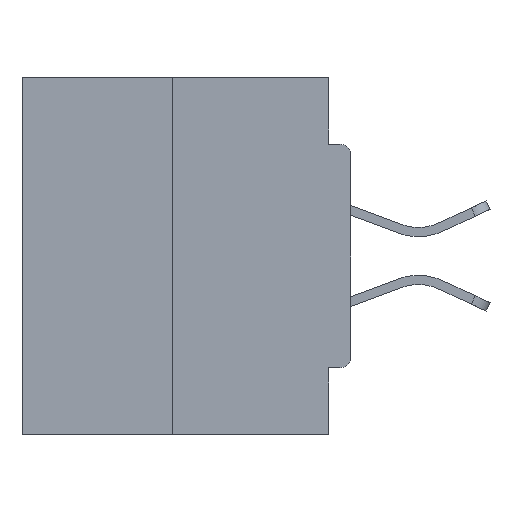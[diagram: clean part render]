
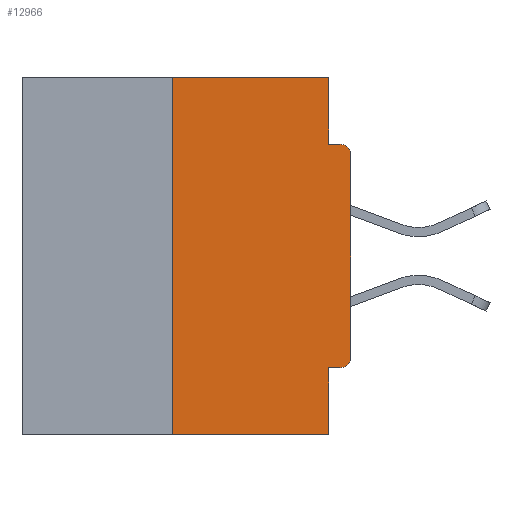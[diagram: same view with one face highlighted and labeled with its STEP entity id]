
A CAD part, left-side view. The second image highlights one B-rep face of the part: STEP entity #12966.
In plain terms, the highlighted planar face has unit normal (-1, 0, 0).
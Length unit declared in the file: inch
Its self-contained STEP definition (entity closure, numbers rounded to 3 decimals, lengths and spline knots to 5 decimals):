
#333 = VECTOR ( 'NONE', #12182, 39.37008 ) ;
#417 = CARTESIAN_POINT ( 'NONE',  ( 0., 0.015, -0.4065 ) ) ;
#547 = CARTESIAN_POINT ( 'NONE',  ( 0., 0., -0.1085 ) ) ;
#563 = EDGE_CURVE ( 'NONE', #22373, #10864, #4484, .T. ) ;
#643 = VERTEX_POINT ( 'NONE', #36403 ) ;
#2013 = VERTEX_POINT ( 'NONE', #417 ) ;
#2313 = CARTESIAN_POINT ( 'NONE',  ( 0., 0.25, 0. ) ) ;
#3175 = LINE ( 'NONE', #6130, #9970 ) ;
#3358 = CIRCLE ( 'NONE', #30537, 0.015 ) ;
#3450 = CARTESIAN_POINT ( 'NONE',  ( 0., 0., 0. ) ) ;
#3706 = EDGE_CURVE ( 'NONE', #19159, #22373, #3175, .T. ) ;
#4159 = VERTEX_POINT ( 'NONE', #19942 ) ;
#4265 = AXIS2_PLACEMENT_3D ( 'NONE', #24446, #10543, #18491 ) ;
#4347 = ORIENTED_EDGE ( 'NONE', *, *, #21684, .F. ) ;
#4484 = LINE ( 'NONE', #18696, #19884 ) ;
#5121 = CARTESIAN_POINT ( 'NONE',  ( 0., 0., -0.3915 ) ) ;
#5281 = DIRECTION ( 'NONE',  ( 0., 0., -1. ) ) ;
#6001 = VECTOR ( 'NONE', #30020, 39.37008 ) ;
#6130 = CARTESIAN_POINT ( 'NONE',  ( 0., 0.031, 0. ) ) ;
#6259 = VERTEX_POINT ( 'NONE', #2313 ) ;
#6501 = VERTEX_POINT ( 'NONE', #547 ) ;
#8288 = DIRECTION ( 'NONE',  ( 1., 0., 0. ) ) ;
#8590 = DIRECTION ( 'NONE',  ( -1., 0., 0. ) ) ;
#9970 = VECTOR ( 'NONE', #28150, 39.37008 ) ;
#10354 = DIRECTION ( 'NONE',  ( 0., -1., 0. ) ) ;
#10543 = DIRECTION ( 'NONE',  ( -1., 0., 0. ) ) ;
#10864 = VERTEX_POINT ( 'NONE', #24368 ) ;
#11917 = VECTOR ( 'NONE', #15080, 39.37008 ) ;
#12182 = DIRECTION ( 'NONE',  ( 0., 1., 0. ) ) ;
#12185 = VERTEX_POINT ( 'NONE', #5121 ) ;
#12966 = ADVANCED_FACE ( 'NONE', ( #22513 ), #30677, .F. ) ;
#13033 = VECTOR ( 'NONE', #10354, 39.37008 ) ;
#13165 = LINE ( 'NONE', #35702, #6001 ) ;
#14017 = CARTESIAN_POINT ( 'NONE',  ( 0., 0.031, 0. ) ) ;
#14531 = EDGE_CURVE ( 'NONE', #4159, #19015, #26332, .T. ) ;
#14701 = LINE ( 'NONE', #3450, #32940 ) ;
#15080 = DIRECTION ( 'NONE',  ( 0., -1., 0. ) ) ;
#15163 = LINE ( 'NONE', #34755, #333 ) ;
#15308 = CARTESIAN_POINT ( 'NONE',  ( 0., 0.031, -0.0935 ) ) ;
#18129 = EDGE_LOOP ( 'NONE', ( #18596, #4347, #33039, #26468, #20094, #22767, #28014, #28565, #25406, #29404 ) ) ;
#18254 = AXIS2_PLACEMENT_3D ( 'NONE', #28437, #8288, #33780 ) ;
#18403 = CARTESIAN_POINT ( 'NONE',  ( 0., 0.46, 0. ) ) ;
#18491 = DIRECTION ( 'NONE',  ( 0., 0., -1. ) ) ;
#18596 = ORIENTED_EDGE ( 'NONE', *, *, #24082, .F. ) ;
#18662 = CARTESIAN_POINT ( 'NONE',  ( 0., 0.031, -0.5 ) ) ;
#18696 = CARTESIAN_POINT ( 'NONE',  ( 0., 0., -0.0935 ) ) ;
#19015 = VERTEX_POINT ( 'NONE', #18662 ) ;
#19159 = VERTEX_POINT ( 'NONE', #14017 ) ;
#19709 = DIRECTION ( 'NONE',  ( 0., 0., 1. ) ) ;
#19884 = VECTOR ( 'NONE', #24459, 39.37008 ) ;
#19942 = CARTESIAN_POINT ( 'NONE',  ( 0., 0.031, -0.4065 ) ) ;
#20094 = ORIENTED_EDGE ( 'NONE', *, *, #33133, .F. ) ;
#20981 = EDGE_CURVE ( 'NONE', #12185, #6501, #14701, .T. ) ;
#21684 = EDGE_CURVE ( 'NONE', #643, #6259, #13165, .T. ) ;
#22123 = EDGE_CURVE ( 'NONE', #643, #19015, #24247, .T. ) ;
#22373 = VERTEX_POINT ( 'NONE', #15308 ) ;
#22513 = FACE_OUTER_BOUND ( 'NONE', #18129, .T. ) ;
#22767 = ORIENTED_EDGE ( 'NONE', *, *, #28122, .T. ) ;
#23977 = LINE ( 'NONE', #18403, #11917 ) ;
#24082 = EDGE_CURVE ( 'NONE', #6259, #19159, #23977, .T. ) ;
#24247 = LINE ( 'NONE', #35663, #13033 ) ;
#24368 = CARTESIAN_POINT ( 'NONE',  ( 0., 0.015, -0.0935 ) ) ;
#24446 = CARTESIAN_POINT ( 'NONE',  ( 0., 0.015, -0.3915 ) ) ;
#24459 = DIRECTION ( 'NONE',  ( 0., -1., 0. ) ) ;
#25406 = ORIENTED_EDGE ( 'NONE', *, *, #563, .F. ) ;
#26332 = LINE ( 'NONE', #35665, #31871 ) ;
#26468 = ORIENTED_EDGE ( 'NONE', *, *, #14531, .F. ) ;
#28014 = ORIENTED_EDGE ( 'NONE', *, *, #20981, .T. ) ;
#28122 = EDGE_CURVE ( 'NONE', #2013, #12185, #30860, .T. ) ;
#28150 = DIRECTION ( 'NONE',  ( 0., 0., -1. ) ) ;
#28437 = CARTESIAN_POINT ( 'NONE',  ( 0., 0.46, 0. ) ) ;
#28565 = ORIENTED_EDGE ( 'NONE', *, *, #32432, .T. ) ;
#28741 = DIRECTION ( 'NONE',  ( 0., 0., -1. ) ) ;
#29404 = ORIENTED_EDGE ( 'NONE', *, *, #3706, .F. ) ;
#30020 = DIRECTION ( 'NONE',  ( 0., 0., 1. ) ) ;
#30537 = AXIS2_PLACEMENT_3D ( 'NONE', #30814, #8590, #5281 ) ;
#30677 = PLANE ( 'NONE',  #18254 ) ;
#30814 = CARTESIAN_POINT ( 'NONE',  ( 0., 0.015, -0.1085 ) ) ;
#30860 = CIRCLE ( 'NONE', #4265, 0.015 ) ;
#31871 = VECTOR ( 'NONE', #28741, 39.37008 ) ;
#32432 = EDGE_CURVE ( 'NONE', #6501, #10864, #3358, .T. ) ;
#32940 = VECTOR ( 'NONE', #19709, 39.37008 ) ;
#33039 = ORIENTED_EDGE ( 'NONE', *, *, #22123, .T. ) ;
#33133 = EDGE_CURVE ( 'NONE', #2013, #4159, #15163, .T. ) ;
#33780 = DIRECTION ( 'NONE',  ( 0., 0., -1. ) ) ;
#34755 = CARTESIAN_POINT ( 'NONE',  ( 0., 0., -0.4065 ) ) ;
#35663 = CARTESIAN_POINT ( 'NONE',  ( 0., 0.46, -0.5 ) ) ;
#35665 = CARTESIAN_POINT ( 'NONE',  ( 0., 0.031, -0.5 ) ) ;
#35702 = CARTESIAN_POINT ( 'NONE',  ( 0., 0.25, 0. ) ) ;
#36403 = CARTESIAN_POINT ( 'NONE',  ( 0., 0.25, -0.5 ) ) ;
